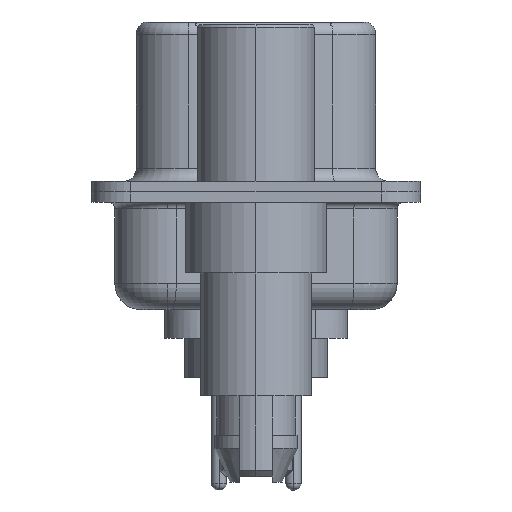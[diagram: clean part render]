
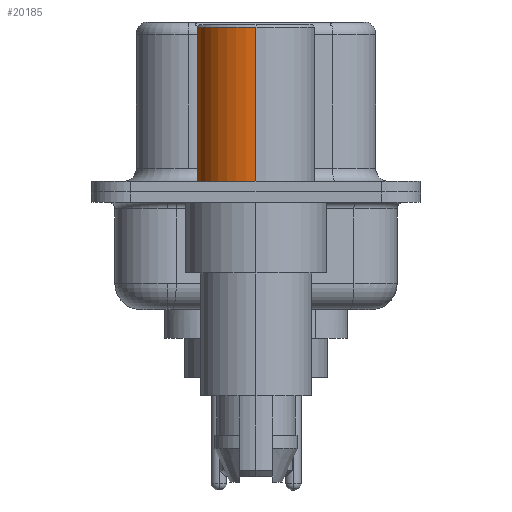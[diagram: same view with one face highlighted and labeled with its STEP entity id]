
A CAD part, left-side view. The second image highlights one B-rep face of the part: STEP entity #20185.
In plain terms, the highlighted cylindrical face has radius 2.25 mm (diameter 4.5 mm), a partial arc.
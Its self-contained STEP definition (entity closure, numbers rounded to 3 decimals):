
#326 = CARTESIAN_POINT ( 'NONE',  ( 0., 0., 0.4 ) ) ;
#330 = DIRECTION ( 'NONE',  ( 0., 0., 1. ) ) ;
#414 = AXIS2_PLACEMENT_3D ( 'NONE', #5760, #2020, #18325 ) ;
#520 = AXIS2_PLACEMENT_3D ( 'NONE', #14759, #3826, #16518 ) ;
#696 = ORIENTED_EDGE ( 'NONE', *, *, #15097, .T. ) ;
#949 = VECTOR ( 'NONE', #330, 1000. ) ;
#2020 = DIRECTION ( 'NONE',  ( 0., 0., 1. ) ) ;
#2109 = LINE ( 'NONE', #9694, #949 ) ;
#2217 = DIRECTION ( 'NONE',  ( 1., 0., 0. ) ) ;
#3424 = VERTEX_POINT ( 'NONE', #10236 ) ;
#3826 = DIRECTION ( 'NONE',  ( 0., 0., 1. ) ) ;
#4067 = CIRCLE ( 'NONE', #18680, 2.25 ) ;
#5310 = EDGE_CURVE ( 'NONE', #7979, #23337, #20805, .T. ) ;
#5430 = FACE_OUTER_BOUND ( 'NONE', #21432, .T. ) ;
#5760 = CARTESIAN_POINT ( 'NONE',  ( 0., 0., 0.581 ) ) ;
#6794 = CARTESIAN_POINT ( 'NONE',  ( 2.25, 0., 6.3 ) ) ;
#7979 = VERTEX_POINT ( 'NONE', #17681 ) ;
#8996 = VERTEX_POINT ( 'NONE', #12382 ) ;
#9694 = CARTESIAN_POINT ( 'NONE',  ( -2.25, 0., 0.581 ) ) ;
#10236 = CARTESIAN_POINT ( 'NONE',  ( -2.25, 0., 6.3 ) ) ;
#10395 = DIRECTION ( 'NONE',  ( 0., 0., 1. ) ) ;
#10577 = VECTOR ( 'NONE', #10395, 1000. ) ;
#10799 = CARTESIAN_POINT ( 'NONE',  ( 2.25, 0., 0.581 ) ) ;
#12382 = CARTESIAN_POINT ( 'NONE',  ( -2.25, 0., 0.4 ) ) ;
#13181 = EDGE_CURVE ( 'NONE', #7979, #8996, #4067, .T. ) ;
#13208 = DIRECTION ( 'NONE',  ( 0., 0., 1. ) ) ;
#13304 = ORIENTED_EDGE ( 'NONE', *, *, #5310, .F. ) ;
#14319 = CIRCLE ( 'NONE', #520, 2.25 ) ;
#14759 = CARTESIAN_POINT ( 'NONE',  ( 0., 0., 6.3 ) ) ;
#15097 = EDGE_CURVE ( 'NONE', #8996, #3424, #2109, .T. ) ;
#16518 = DIRECTION ( 'NONE',  ( 1., 0., 0. ) ) ;
#17398 = EDGE_CURVE ( 'NONE', #23337, #3424, #14319, .T. ) ;
#17681 = CARTESIAN_POINT ( 'NONE',  ( 2.25, 0., 0.4 ) ) ;
#18325 = DIRECTION ( 'NONE',  ( 1., 0., 0. ) ) ;
#18680 = AXIS2_PLACEMENT_3D ( 'NONE', #326, #13208, #2217 ) ;
#19210 = CYLINDRICAL_SURFACE ( 'NONE', #414, 2.25 ) ;
#19290 = ORIENTED_EDGE ( 'NONE', *, *, #13181, .T. ) ;
#20185 = ADVANCED_FACE ( 'NONE', ( #5430 ), #19210, .T. ) ;
#20355 = ORIENTED_EDGE ( 'NONE', *, *, #17398, .F. ) ;
#20805 = LINE ( 'NONE', #10799, #10577 ) ;
#21432 = EDGE_LOOP ( 'NONE', ( #19290, #696, #20355, #13304 ) ) ;
#23337 = VERTEX_POINT ( 'NONE', #6794 ) ;
